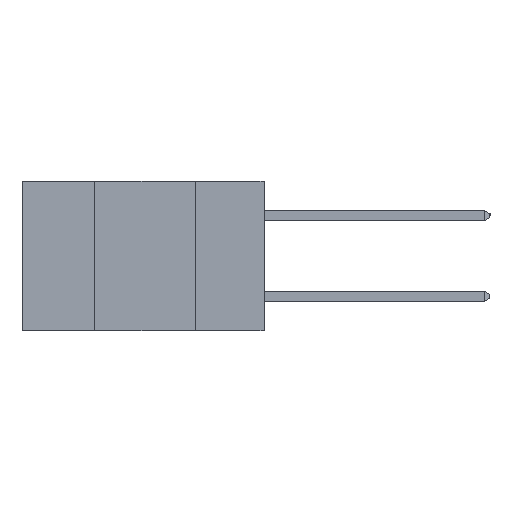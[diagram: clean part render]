
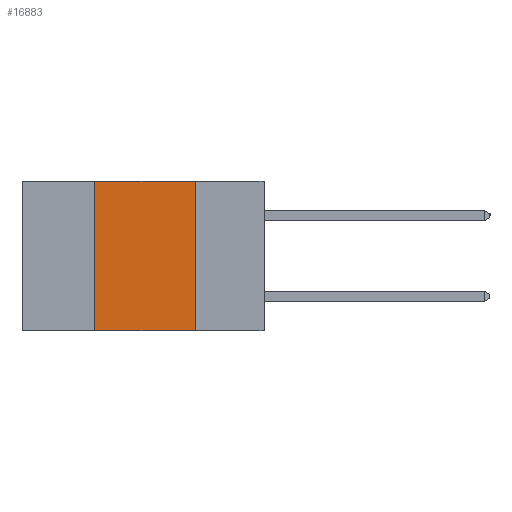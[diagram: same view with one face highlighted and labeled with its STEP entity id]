
A CAD part, left-side view. The second image highlights one B-rep face of the part: STEP entity #16883.
In plain terms, the highlighted planar face has unit normal (-1, 0, 0).
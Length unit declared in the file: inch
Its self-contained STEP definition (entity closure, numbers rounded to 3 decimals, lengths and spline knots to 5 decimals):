
#239 = VECTOR ( 'NONE', #17283, 39.37008 ) ;
#742 = EDGE_LOOP ( 'NONE', ( #5761, #9818, #19645, #15162 ) ) ;
#1735 = VECTOR ( 'NONE', #5612, 39.37008 ) ;
#2718 = CARTESIAN_POINT ( 'NONE',  ( 0., 0.42, 0. ) ) ;
#3195 = AXIS2_PLACEMENT_3D ( 'NONE', #20349, #3977, #5896 ) ;
#3977 = DIRECTION ( 'NONE',  ( 1., 0., 0. ) ) ;
#4927 = CARTESIAN_POINT ( 'NONE',  ( 0., 0.42, -0.37 ) ) ;
#4929 = LINE ( 'NONE', #15839, #1735 ) ;
#5612 = DIRECTION ( 'NONE',  ( 0., -1., 0. ) ) ;
#5761 = ORIENTED_EDGE ( 'NONE', *, *, #19573, .F. ) ;
#5896 = DIRECTION ( 'NONE',  ( 0., 0., -1. ) ) ;
#9112 = VERTEX_POINT ( 'NONE', #12036 ) ;
#9399 = CARTESIAN_POINT ( 'NONE',  ( 0., 0.42, -0.37 ) ) ;
#9738 = LINE ( 'NONE', #13322, #239 ) ;
#9818 = ORIENTED_EDGE ( 'NONE', *, *, #23228, .F. ) ;
#10232 = CARTESIAN_POINT ( 'NONE',  ( 0., 0.17, -0.37 ) ) ;
#10348 = DIRECTION ( 'NONE',  ( 0., 0., -1. ) ) ;
#12036 = CARTESIAN_POINT ( 'NONE',  ( 0., 0.17, -0.37 ) ) ;
#12163 = LINE ( 'NONE', #10232, #15936 ) ;
#13322 = CARTESIAN_POINT ( 'NONE',  ( 0., 0.6, -0.37 ) ) ;
#14260 = VERTEX_POINT ( 'NONE', #20837 ) ;
#15162 = ORIENTED_EDGE ( 'NONE', *, *, #19887, .T. ) ;
#15596 = VECTOR ( 'NONE', #16724, 39.37008 ) ;
#15839 = CARTESIAN_POINT ( 'NONE',  ( 0., 0.6, 0. ) ) ;
#15936 = VECTOR ( 'NONE', #10348, 39.37008 ) ;
#16724 = DIRECTION ( 'NONE',  ( 0., 0., 1. ) ) ;
#16883 = ADVANCED_FACE ( 'NONE', ( #20601 ), #16928, .F. ) ;
#16928 = PLANE ( 'NONE',  #3195 ) ;
#17062 = VERTEX_POINT ( 'NONE', #4927 ) ;
#17283 = DIRECTION ( 'NONE',  ( 0., -1., 0. ) ) ;
#18495 = LINE ( 'NONE', #9399, #15596 ) ;
#19573 = EDGE_CURVE ( 'NONE', #14260, #9112, #12163, .T. ) ;
#19645 = ORIENTED_EDGE ( 'NONE', *, *, #21269, .F. ) ;
#19887 = EDGE_CURVE ( 'NONE', #17062, #9112, #9738, .T. ) ;
#20349 = CARTESIAN_POINT ( 'NONE',  ( 0., 0.6, 0. ) ) ;
#20601 = FACE_OUTER_BOUND ( 'NONE', #742, .T. ) ;
#20825 = VERTEX_POINT ( 'NONE', #2718 ) ;
#20837 = CARTESIAN_POINT ( 'NONE',  ( 0., 0.17, 0. ) ) ;
#21269 = EDGE_CURVE ( 'NONE', #17062, #20825, #18495, .T. ) ;
#23228 = EDGE_CURVE ( 'NONE', #20825, #14260, #4929, .T. ) ;
